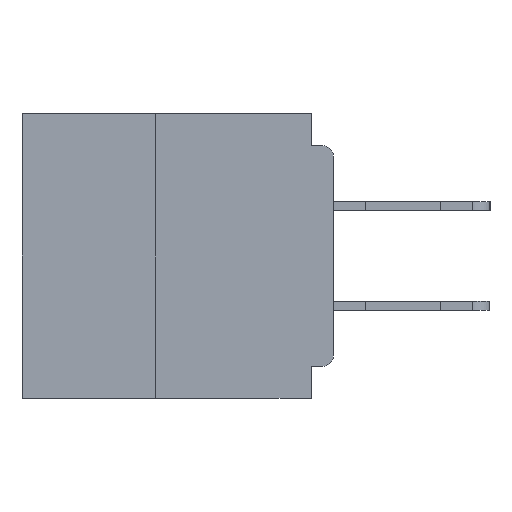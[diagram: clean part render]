
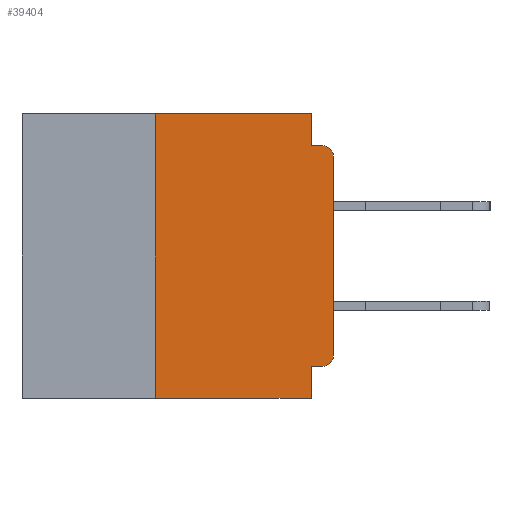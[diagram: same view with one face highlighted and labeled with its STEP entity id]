
A CAD part, left-side view. The second image highlights one B-rep face of the part: STEP entity #39404.
In plain terms, the highlighted planar face has unit normal (-1, 0, 0).
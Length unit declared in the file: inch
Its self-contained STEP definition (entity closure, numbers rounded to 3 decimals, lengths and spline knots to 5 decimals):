
#639 = DIRECTION ( 'NONE',  ( 1., 0., 0. ) ) ;
#1222 = VECTOR ( 'NONE', #3238, 39.37008 ) ;
#1488 = VECTOR ( 'NONE', #11988, 39.37008 ) ;
#1886 = CIRCLE ( 'NONE', #6104, 0.015 ) ;
#2369 = VECTOR ( 'NONE', #22280, 39.37008 ) ;
#2475 = EDGE_CURVE ( 'NONE', #16528, #34470, #20432, .T. ) ;
#2571 = FACE_OUTER_BOUND ( 'NONE', #13770, .T. ) ;
#3238 = DIRECTION ( 'NONE',  ( 0., 0., 1. ) ) ;
#3505 = LINE ( 'NONE', #7556, #23742 ) ;
#4726 = CARTESIAN_POINT ( 'NONE',  ( 0., 0.015, -0.34 ) ) ;
#4769 = VECTOR ( 'NONE', #11499, 39.37008 ) ;
#5034 = EDGE_CURVE ( 'NONE', #26011, #37826, #1886, .T. ) ;
#6104 = AXIS2_PLACEMENT_3D ( 'NONE', #30670, #30627, #30582 ) ;
#7027 = ORIENTED_EDGE ( 'NONE', *, *, #24233, .T. ) ;
#7556 = CARTESIAN_POINT ( 'NONE',  ( 0., 0.25, -0.4 ) ) ;
#8141 = DIRECTION ( 'NONE',  ( 0., 0., -1. ) ) ;
#8896 = DIRECTION ( 'NONE',  ( 0., -1., 0. ) ) ;
#9694 = ORIENTED_EDGE ( 'NONE', *, *, #43318, .F. ) ;
#10516 = LINE ( 'NONE', #35645, #1488 ) ;
#11499 = DIRECTION ( 'NONE',  ( 0., -1., 0. ) ) ;
#11530 = CARTESIAN_POINT ( 'NONE',  ( 0., 0.031, -0.355 ) ) ;
#11984 = LINE ( 'NONE', #20025, #37862 ) ;
#11988 = DIRECTION ( 'NONE',  ( 0., 1., 0. ) ) ;
#12238 = CARTESIAN_POINT ( 'NONE',  ( 0., 0.031, 0. ) ) ;
#12894 = ORIENTED_EDGE ( 'NONE', *, *, #2475, .F. ) ;
#13559 = AXIS2_PLACEMENT_3D ( 'NONE', #17439, #639, #24453 ) ;
#13770 = EDGE_LOOP ( 'NONE', ( #20578, #14144, #32145, #27400, #36349, #9694, #19798, #12894, #30865, #7027 ) ) ;
#13939 = EDGE_CURVE ( 'NONE', #16139, #22612, #33376, .T. ) ;
#14144 = ORIENTED_EDGE ( 'NONE', *, *, #5034, .T. ) ;
#14314 = VERTEX_POINT ( 'NONE', #29329 ) ;
#16139 = VERTEX_POINT ( 'NONE', #23019 ) ;
#16528 = VERTEX_POINT ( 'NONE', #11530 ) ;
#16827 = VERTEX_POINT ( 'NONE', #26784 ) ;
#17439 = CARTESIAN_POINT ( 'NONE',  ( 0., 0.437, 0. ) ) ;
#17498 = CARTESIAN_POINT ( 'NONE',  ( 0., 0., 0. ) ) ;
#19798 = ORIENTED_EDGE ( 'NONE', *, *, #28262, .T. ) ;
#20025 = CARTESIAN_POINT ( 'NONE',  ( 0., 0.437, 0. ) ) ;
#20301 = AXIS2_PLACEMENT_3D ( 'NONE', #4726, #28455, #8141 ) ;
#20432 = LINE ( 'NONE', #36447, #2369 ) ;
#20578 = ORIENTED_EDGE ( 'NONE', *, *, #32044, .T. ) ;
#22280 = DIRECTION ( 'NONE',  ( 0., 0., -1. ) ) ;
#22612 = VERTEX_POINT ( 'NONE', #31239 ) ;
#23019 = CARTESIAN_POINT ( 'NONE',  ( 0., 0.031, 0. ) ) ;
#23084 = VERTEX_POINT ( 'NONE', #42000 ) ;
#23424 = CARTESIAN_POINT ( 'NONE',  ( 0., 0.031, -0.4 ) ) ;
#23742 = VECTOR ( 'NONE', #24522, 39.37008 ) ;
#24233 = EDGE_CURVE ( 'NONE', #23084, #14314, #42321, .T. ) ;
#24447 = VECTOR ( 'NONE', #42561, 39.37008 ) ;
#24453 = DIRECTION ( 'NONE',  ( 0., 0., -1. ) ) ;
#24522 = DIRECTION ( 'NONE',  ( 0., 0., 1. ) ) ;
#25616 = CARTESIAN_POINT ( 'NONE',  ( 0., 0.015, -0.045 ) ) ;
#25930 = EDGE_CURVE ( 'NONE', #23084, #16528, #10516, .T. ) ;
#26011 = VERTEX_POINT ( 'NONE', #39278 ) ;
#26784 = CARTESIAN_POINT ( 'NONE',  ( 0., 0.25, -0.4 ) ) ;
#27395 = EDGE_CURVE ( 'NONE', #41659, #16139, #11984, .T. ) ;
#27400 = ORIENTED_EDGE ( 'NONE', *, *, #13939, .F. ) ;
#28262 = EDGE_CURVE ( 'NONE', #16827, #34470, #40690, .T. ) ;
#28398 = CARTESIAN_POINT ( 'NONE',  ( 0., 0.437, -0.4 ) ) ;
#28455 = DIRECTION ( 'NONE',  ( -1., 0., 0. ) ) ;
#29329 = CARTESIAN_POINT ( 'NONE',  ( 0., 0., -0.34 ) ) ;
#30582 = DIRECTION ( 'NONE',  ( 0., 0., -1. ) ) ;
#30627 = DIRECTION ( 'NONE',  ( -1., 0., 0. ) ) ;
#30670 = CARTESIAN_POINT ( 'NONE',  ( 0., 0.015, -0.06 ) ) ;
#30865 = ORIENTED_EDGE ( 'NONE', *, *, #25930, .F. ) ;
#30870 = CARTESIAN_POINT ( 'NONE',  ( 0., 0.25, 0. ) ) ;
#30929 = VECTOR ( 'NONE', #8896, 39.37008 ) ;
#31239 = CARTESIAN_POINT ( 'NONE',  ( 0., 0.031, -0.045 ) ) ;
#32044 = EDGE_CURVE ( 'NONE', #14314, #26011, #37236, .T. ) ;
#32145 = ORIENTED_EDGE ( 'NONE', *, *, #35725, .F. ) ;
#32590 = CARTESIAN_POINT ( 'NONE',  ( 0., 0., -0.045 ) ) ;
#33376 = LINE ( 'NONE', #12238, #24447 ) ;
#34470 = VERTEX_POINT ( 'NONE', #23424 ) ;
#35645 = CARTESIAN_POINT ( 'NONE',  ( 0., 0., -0.355 ) ) ;
#35725 = EDGE_CURVE ( 'NONE', #22612, #37826, #38822, .T. ) ;
#36349 = ORIENTED_EDGE ( 'NONE', *, *, #27395, .F. ) ;
#36447 = CARTESIAN_POINT ( 'NONE',  ( 0., 0.031, -0.4 ) ) ;
#37236 = LINE ( 'NONE', #17498, #1222 ) ;
#37826 = VERTEX_POINT ( 'NONE', #25616 ) ;
#37862 = VECTOR ( 'NONE', #40192, 39.37008 ) ;
#38822 = LINE ( 'NONE', #32590, #30929 ) ;
#39278 = CARTESIAN_POINT ( 'NONE',  ( 0., 0., -0.06 ) ) ;
#39404 = ADVANCED_FACE ( 'NONE', ( #2571 ), #41112, .F. ) ;
#40192 = DIRECTION ( 'NONE',  ( 0., -1., 0. ) ) ;
#40690 = LINE ( 'NONE', #28398, #4769 ) ;
#41112 = PLANE ( 'NONE',  #13559 ) ;
#41659 = VERTEX_POINT ( 'NONE', #30870 ) ;
#42000 = CARTESIAN_POINT ( 'NONE',  ( 0., 0.015, -0.355 ) ) ;
#42321 = CIRCLE ( 'NONE', #20301, 0.015 ) ;
#42561 = DIRECTION ( 'NONE',  ( 0., 0., -1. ) ) ;
#43318 = EDGE_CURVE ( 'NONE', #16827, #41659, #3505, .T. ) ;
